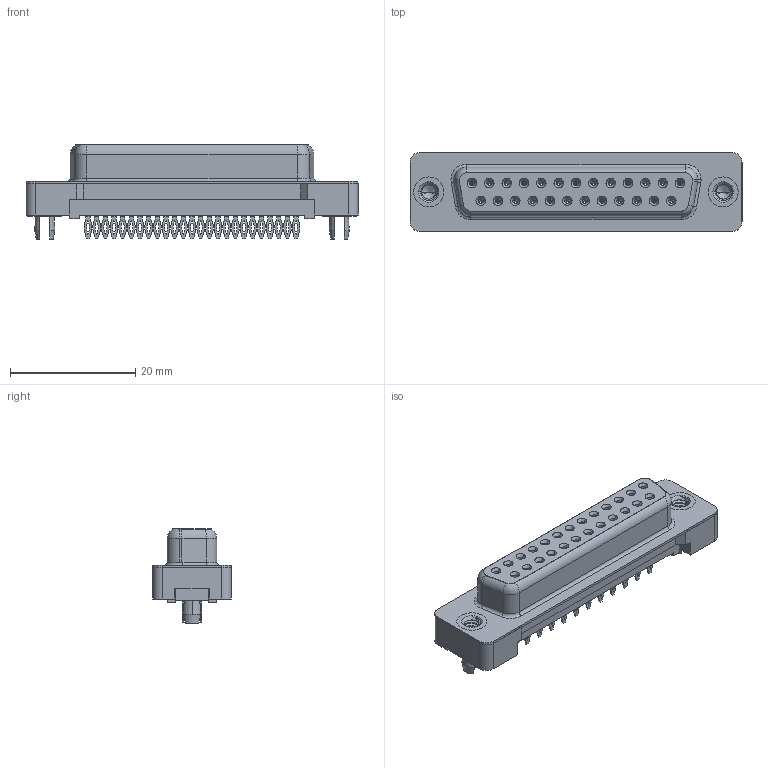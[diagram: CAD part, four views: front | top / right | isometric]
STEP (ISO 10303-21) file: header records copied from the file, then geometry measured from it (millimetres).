
FILE_DESCRIPTION (( 'STEP AP203' ), '1' );
FILE_NAME ('628-025-226-016.STEP', '2020-07-15T23:50:49', ( '' ), ( '' ), 'SwSTEP 2.0', 'SolidWorks 2020', '' );
FILE_SCHEMA (( 'CONFIG_CONTROL_DESIGN' ));
Length unit declared in the file: millimetre
Products named in the file (6): 628-025-226-016; 628 PB Shell_25 Contacts; 628 PB 4-40 Threaded Rivet with Boardlock; 628 PB Contact Row 1_26; 628 PB Contact Row 2_26; 628 Plastic Body Housing_25 Contacts
Assembly tree (29 placements, depth 2):
  628-025-226-016
    628 Plastic Body Housing_25 Contacts
    628 PB Shell_25 Contacts
    628 PB Contact Row 1_26  x13
    628 PB Contact Row 2_26  x12
    628 PB 4-40 Threaded Rivet with Boardlock  x2
Bounding box: 53.05 x 12.55 x 15.05 mm (x, y, z)
Volume: 3317.6 mm3; surface area: 8562.7 mm2
Topology: 29 solids, 29 shells, 2511 faces, 6131 edges, 3716 vertices
Faces by surface type: plane 1034, cylinder 598, bspline 556, torus 176, cone 147
Entity records: 21598 total; most frequent: CARTESIAN_POINT 6117, ORIENTED_EDGE 2964, DIRECTION 2875, EDGE_CURVE 1482, AXIS2_PLACEMENT_3D 985, VERTEX_POINT 927, VECTOR 905, LINE 905
